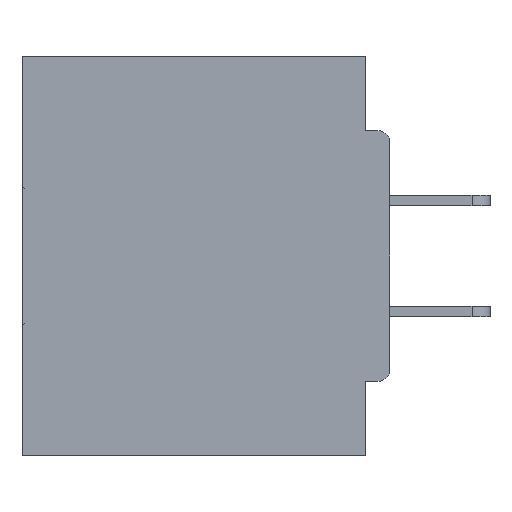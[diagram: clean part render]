
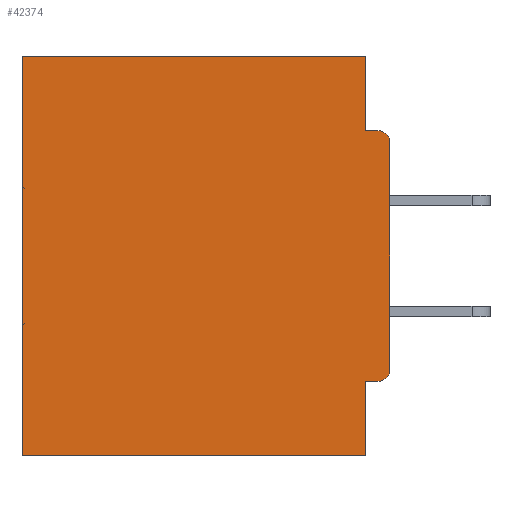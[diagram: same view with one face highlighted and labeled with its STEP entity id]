
A CAD part, left-side view. The second image highlights one B-rep face of the part: STEP entity #42374.
In plain terms, the highlighted planar face has unit normal (-1, 0, 0).
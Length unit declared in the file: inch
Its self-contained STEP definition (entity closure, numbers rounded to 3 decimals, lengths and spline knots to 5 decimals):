
#401 = ORIENTED_EDGE ( 'NONE', *, *, #29212, .F. ) ;
#717 = EDGE_CURVE ( 'NONE', #13697, #34085, #23158, .T. ) ;
#922 = ORIENTED_EDGE ( 'NONE', *, *, #30668, .F. ) ;
#1409 = DIRECTION ( 'NONE',  ( 0., 1., 0. ) ) ;
#1780 = DIRECTION ( 'NONE',  ( 0., 1., 0. ) ) ;
#2551 = VERTEX_POINT ( 'NONE', #7398 ) ;
#3509 = DIRECTION ( 'NONE',  ( 0., 0., -1. ) ) ;
#3733 = EDGE_CURVE ( 'NONE', #31355, #15625, #27319, .T. ) ;
#5150 = CARTESIAN_POINT ( 'NONE',  ( 0.298, 0.031, -0.0935 ) ) ;
#5851 = CARTESIAN_POINT ( 'NONE',  ( 0.298, 0.031, -0.4065 ) ) ;
#6168 = VECTOR ( 'NONE', #1780, 39.37008 ) ;
#6479 = VERTEX_POINT ( 'NONE', #5150 ) ;
#6946 = DIRECTION ( 'NONE',  ( 0., 0., -1. ) ) ;
#7398 = CARTESIAN_POINT ( 'NONE',  ( 0.298, 0.015, -0.0935 ) ) ;
#7405 = DIRECTION ( 'NONE',  ( 1., 0., 0. ) ) ;
#8820 = DIRECTION ( 'NONE',  ( 0., 0., -1. ) ) ;
#10908 = DIRECTION ( 'NONE',  ( 0., 0., -1. ) ) ;
#11519 = AXIS2_PLACEMENT_3D ( 'NONE', #40987, #7405, #3509 ) ;
#11628 = CARTESIAN_POINT ( 'NONE',  ( 0.298, 0.031, -0.5 ) ) ;
#12058 = ORIENTED_EDGE ( 'NONE', *, *, #42448, .T. ) ;
#12256 = CARTESIAN_POINT ( 'NONE',  ( 0.298, 0., -0.3915 ) ) ;
#12441 = VECTOR ( 'NONE', #17098, 39.37008 ) ;
#13070 = ORIENTED_EDGE ( 'NONE', *, *, #19338, .T. ) ;
#13071 = VECTOR ( 'NONE', #25402, 39.37008 ) ;
#13322 = DIRECTION ( 'NONE',  ( 0., -1., 0. ) ) ;
#13697 = VERTEX_POINT ( 'NONE', #19319 ) ;
#13779 = VECTOR ( 'NONE', #31379, 39.37008 ) ;
#13783 = LINE ( 'NONE', #20978, #38303 ) ;
#14377 = VECTOR ( 'NONE', #13322, 39.37008 ) ;
#15497 = CARTESIAN_POINT ( 'NONE',  ( 0.298, 0.015, -0.1085 ) ) ;
#15625 = VERTEX_POINT ( 'NONE', #12256 ) ;
#16743 = CARTESIAN_POINT ( 'NONE',  ( 0.298, 0.46, -0.5 ) ) ;
#16794 = ORIENTED_EDGE ( 'NONE', *, *, #29247, .T. ) ;
#17098 = DIRECTION ( 'NONE',  ( 0., 0., -1. ) ) ;
#19319 = CARTESIAN_POINT ( 'NONE',  ( 0.298, 0.46, 0. ) ) ;
#19338 = EDGE_CURVE ( 'NONE', #19743, #13697, #40766, .T. ) ;
#19743 = VERTEX_POINT ( 'NONE', #27815 ) ;
#20568 = CARTESIAN_POINT ( 'NONE',  ( 0.298, 0.015, -0.4065 ) ) ;
#20978 = CARTESIAN_POINT ( 'NONE',  ( 0.298, 0.031, -0.5 ) ) ;
#21752 = CARTESIAN_POINT ( 'NONE',  ( 0.298, 0., -0.5 ) ) ;
#22240 = CARTESIAN_POINT ( 'NONE',  ( 0.298, 0., 0. ) ) ;
#22292 = LINE ( 'NONE', #11628, #13779 ) ;
#22810 = VERTEX_POINT ( 'NONE', #20568 ) ;
#23158 = LINE ( 'NONE', #42377, #13071 ) ;
#23379 = LINE ( 'NONE', #43841, #14377 ) ;
#23873 = CARTESIAN_POINT ( 'NONE',  ( 0.298, 0.015, -0.3915 ) ) ;
#24322 = PLANE ( 'NONE',  #11519 ) ;
#24576 = AXIS2_PLACEMENT_3D ( 'NONE', #15497, #39582, #8820 ) ;
#24701 = CARTESIAN_POINT ( 'NONE',  ( 0.298, 0., 0. ) ) ;
#24968 = LINE ( 'NONE', #35215, #31896 ) ;
#25150 = CIRCLE ( 'NONE', #24576, 0.015 ) ;
#25170 = AXIS2_PLACEMENT_3D ( 'NONE', #23873, #41292, #6946 ) ;
#25260 = CARTESIAN_POINT ( 'NONE',  ( 0.298, 0., -0.1085 ) ) ;
#25402 = DIRECTION ( 'NONE',  ( 0., 0., -1. ) ) ;
#26686 = EDGE_LOOP ( 'NONE', ( #16794, #39740, #922, #13070, #35734, #401, #42835, #27118, #12058, #38845 ) ) ;
#27118 = ORIENTED_EDGE ( 'NONE', *, *, #42529, .F. ) ;
#27319 = LINE ( 'NONE', #24701, #12441 ) ;
#27815 = CARTESIAN_POINT ( 'NONE',  ( 0.298, 0.031, 0. ) ) ;
#28232 = DIRECTION ( 'NONE',  ( 0., 1., 0. ) ) ;
#29212 = EDGE_CURVE ( 'NONE', #43648, #34085, #37919, .T. ) ;
#29247 = EDGE_CURVE ( 'NONE', #31355, #2551, #25150, .T. ) ;
#30668 = EDGE_CURVE ( 'NONE', #19743, #6479, #13783, .T. ) ;
#31355 = VERTEX_POINT ( 'NONE', #25260 ) ;
#31379 = DIRECTION ( 'NONE',  ( 0., 0., -1. ) ) ;
#31896 = VECTOR ( 'NONE', #28232, 39.37008 ) ;
#34085 = VERTEX_POINT ( 'NONE', #16743 ) ;
#35215 = CARTESIAN_POINT ( 'NONE',  ( 0.298, 0., -0.4065 ) ) ;
#35734 = ORIENTED_EDGE ( 'NONE', *, *, #717, .T. ) ;
#37099 = EDGE_CURVE ( 'NONE', #6479, #2551, #23379, .T. ) ;
#37454 = VERTEX_POINT ( 'NONE', #5851 ) ;
#37919 = LINE ( 'NONE', #21752, #42710 ) ;
#38069 = CARTESIAN_POINT ( 'NONE',  ( 0.298, 0.031, -0.5 ) ) ;
#38277 = EDGE_CURVE ( 'NONE', #37454, #43648, #22292, .T. ) ;
#38303 = VECTOR ( 'NONE', #10908, 39.37008 ) ;
#38845 = ORIENTED_EDGE ( 'NONE', *, *, #3733, .F. ) ;
#39582 = DIRECTION ( 'NONE',  ( -1., 0., 0. ) ) ;
#39740 = ORIENTED_EDGE ( 'NONE', *, *, #37099, .F. ) ;
#39851 = CIRCLE ( 'NONE', #25170, 0.015 ) ;
#40766 = LINE ( 'NONE', #22240, #6168 ) ;
#40924 = FACE_OUTER_BOUND ( 'NONE', #26686, .T. ) ;
#40987 = CARTESIAN_POINT ( 'NONE',  ( 0.298, 0., 0. ) ) ;
#41292 = DIRECTION ( 'NONE',  ( -1., 0., 0. ) ) ;
#42374 = ADVANCED_FACE ( 'NONE', ( #40924 ), #24322, .F. ) ;
#42377 = CARTESIAN_POINT ( 'NONE',  ( 0.298, 0.46, 0. ) ) ;
#42448 = EDGE_CURVE ( 'NONE', #22810, #15625, #39851, .T. ) ;
#42529 = EDGE_CURVE ( 'NONE', #22810, #37454, #24968, .T. ) ;
#42710 = VECTOR ( 'NONE', #1409, 39.37008 ) ;
#42835 = ORIENTED_EDGE ( 'NONE', *, *, #38277, .F. ) ;
#43648 = VERTEX_POINT ( 'NONE', #38069 ) ;
#43841 = CARTESIAN_POINT ( 'NONE',  ( 0.298, 0., -0.0935 ) ) ;
